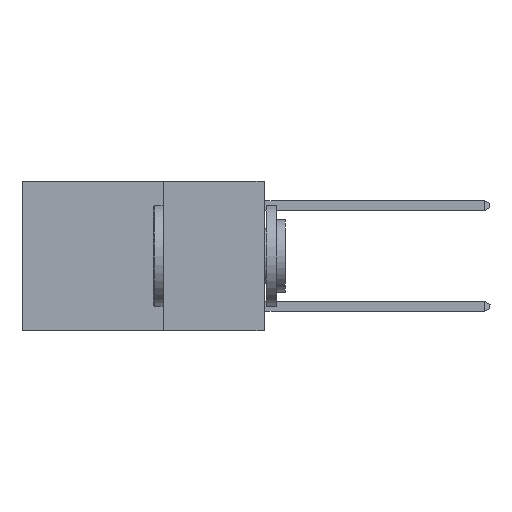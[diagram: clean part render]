
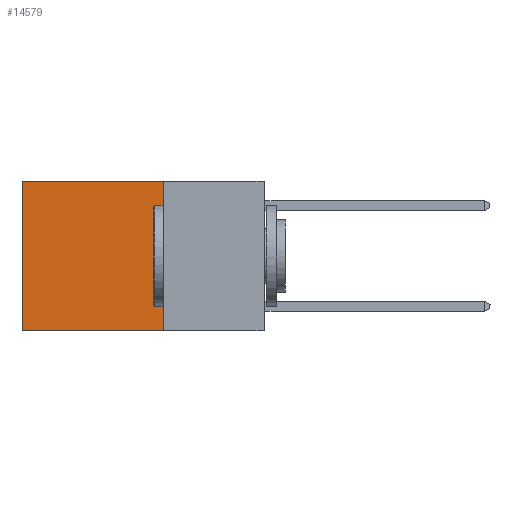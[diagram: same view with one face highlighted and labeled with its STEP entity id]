
A CAD part, left-side view. The second image highlights one B-rep face of the part: STEP entity #14579.
In plain terms, the highlighted planar face has unit normal (-1, 0, 0).
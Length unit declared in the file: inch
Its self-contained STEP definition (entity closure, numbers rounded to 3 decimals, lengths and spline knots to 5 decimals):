
#535 = EDGE_CURVE ( 'NONE', #17649, #8741, #5950, .T. ) ;
#627 = EDGE_CURVE ( 'NONE', #17649, #4103, #21067, .T. ) ;
#681 = CARTESIAN_POINT ( 'NONE',  ( 0.2625, 0.6, 0. ) ) ;
#743 = CARTESIAN_POINT ( 'NONE',  ( 0.2625, 0.25, -0.37 ) ) ;
#2751 = ORIENTED_EDGE ( 'NONE', *, *, #627, .T. ) ;
#3860 = DIRECTION ( 'NONE',  ( 0., 0., -1. ) ) ;
#3943 = VECTOR ( 'NONE', #3860, 39.37008 ) ;
#4103 = VERTEX_POINT ( 'NONE', #681 ) ;
#4964 = EDGE_CURVE ( 'NONE', #4103, #20525, #11964, .T. ) ;
#5185 = VECTOR ( 'NONE', #25118, 39.37008 ) ;
#5270 = VECTOR ( 'NONE', #26942, 39.37008 ) ;
#5950 = LINE ( 'NONE', #8256, #5185 ) ;
#6110 = CARTESIAN_POINT ( 'NONE',  ( 0.2625, 0.25, 0. ) ) ;
#6330 = ORIENTED_EDGE ( 'NONE', *, *, #535, .F. ) ;
#7459 = CARTESIAN_POINT ( 'NONE',  ( 0.2625, 0.6, -0.37 ) ) ;
#8041 = EDGE_LOOP ( 'NONE', ( #25301, #18084, #6330, #2751 ) ) ;
#8256 = CARTESIAN_POINT ( 'NONE',  ( 0.2625, 0.25, 0. ) ) ;
#8741 = VERTEX_POINT ( 'NONE', #743 ) ;
#11462 = CARTESIAN_POINT ( 'NONE',  ( 0.2625, 0.25, 0. ) ) ;
#11732 = DIRECTION ( 'NONE',  ( 1., 0., 0. ) ) ;
#11758 = AXIS2_PLACEMENT_3D ( 'NONE', #30765, #11732, #28490 ) ;
#11964 = LINE ( 'NONE', #15999, #3943 ) ;
#14579 = ADVANCED_FACE ( 'NONE', ( #25657 ), #26139, .F. ) ;
#14767 = EDGE_CURVE ( 'NONE', #8741, #20525, #18932, .T. ) ;
#15999 = CARTESIAN_POINT ( 'NONE',  ( 0.2625, 0.6, 0. ) ) ;
#17649 = VERTEX_POINT ( 'NONE', #11462 ) ;
#18084 = ORIENTED_EDGE ( 'NONE', *, *, #14767, .F. ) ;
#18206 = DIRECTION ( 'NONE',  ( 0., 1., 0. ) ) ;
#18932 = LINE ( 'NONE', #24538, #5270 ) ;
#20525 = VERTEX_POINT ( 'NONE', #7459 ) ;
#21067 = LINE ( 'NONE', #6110, #27417 ) ;
#24538 = CARTESIAN_POINT ( 'NONE',  ( 0.2625, 0.25, -0.37 ) ) ;
#25118 = DIRECTION ( 'NONE',  ( 0., 0., -1. ) ) ;
#25301 = ORIENTED_EDGE ( 'NONE', *, *, #4964, .T. ) ;
#25657 = FACE_OUTER_BOUND ( 'NONE', #8041, .T. ) ;
#26139 = PLANE ( 'NONE',  #11758 ) ;
#26942 = DIRECTION ( 'NONE',  ( 0., 1., 0. ) ) ;
#27417 = VECTOR ( 'NONE', #18206, 39.37008 ) ;
#28490 = DIRECTION ( 'NONE',  ( 0., 0., -1. ) ) ;
#30765 = CARTESIAN_POINT ( 'NONE',  ( 0.2625, 0.25, 0. ) ) ;
